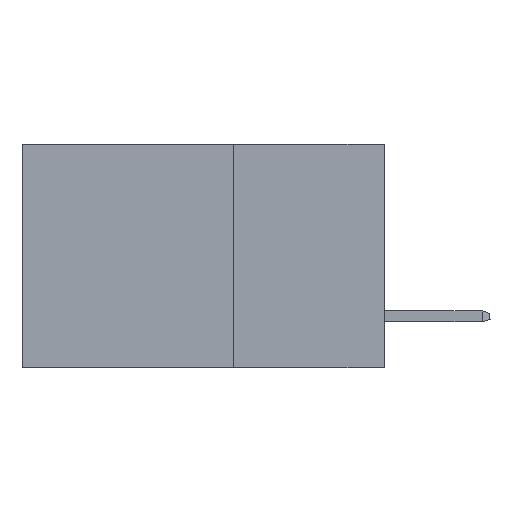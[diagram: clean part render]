
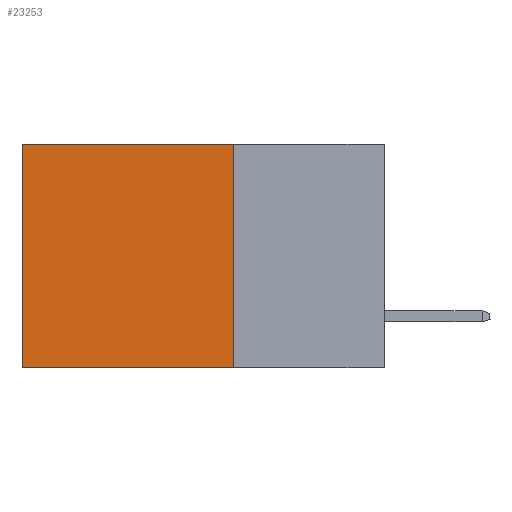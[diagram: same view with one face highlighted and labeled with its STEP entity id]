
A CAD part, left-side view. The second image highlights one B-rep face of the part: STEP entity #23253.
In plain terms, the highlighted planar face has unit normal (-1, 0, 0).
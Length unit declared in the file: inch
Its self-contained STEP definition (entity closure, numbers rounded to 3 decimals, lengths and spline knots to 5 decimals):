
#856 = CARTESIAN_POINT ( 'NONE',  ( 0.298, 0.6, 0. ) ) ;
#1150 = FACE_OUTER_BOUND ( 'NONE', #5787, .T. ) ;
#1282 = AXIS2_PLACEMENT_3D ( 'NONE', #12251, #8460, #14535 ) ;
#1731 = LINE ( 'NONE', #18426, #20809 ) ;
#4433 = VECTOR ( 'NONE', #16250, 39.37008 ) ;
#5022 = CARTESIAN_POINT ( 'NONE',  ( 0.298, 0.25, 0. ) ) ;
#5787 = EDGE_LOOP ( 'NONE', ( #23799, #16752, #11479, #19710 ) ) ;
#6522 = DIRECTION ( 'NONE',  ( 0., 0., -1. ) ) ;
#7714 = CARTESIAN_POINT ( 'NONE',  ( 0.298, 0.6, 0. ) ) ;
#8460 = DIRECTION ( 'NONE',  ( 1., 0., 0. ) ) ;
#8513 = LINE ( 'NONE', #856, #18653 ) ;
#8552 = VERTEX_POINT ( 'NONE', #15728 ) ;
#10761 = LINE ( 'NONE', #5022, #4433 ) ;
#11085 = CARTESIAN_POINT ( 'NONE',  ( 0.298, 0.25, 0. ) ) ;
#11275 = DIRECTION ( 'NONE',  ( 0., 0., -1. ) ) ;
#11479 = ORIENTED_EDGE ( 'NONE', *, *, #13270, .F. ) ;
#12226 = EDGE_CURVE ( 'NONE', #18486, #8552, #1731, .T. ) ;
#12251 = CARTESIAN_POINT ( 'NONE',  ( 0.298, 0.25, 0. ) ) ;
#12773 = VERTEX_POINT ( 'NONE', #7714 ) ;
#13270 = EDGE_CURVE ( 'NONE', #23477, #18486, #20190, .T. ) ;
#13540 = VECTOR ( 'NONE', #11275, 39.37008 ) ;
#14206 = PLANE ( 'NONE',  #1282 ) ;
#14535 = DIRECTION ( 'NONE',  ( 0., 0., -1. ) ) ;
#15475 = EDGE_CURVE ( 'NONE', #12773, #8552, #8513, .T. ) ;
#15728 = CARTESIAN_POINT ( 'NONE',  ( 0.298, 0.6, -0.37 ) ) ;
#16250 = DIRECTION ( 'NONE',  ( 0., 1., 0. ) ) ;
#16588 = DIRECTION ( 'NONE',  ( 0., 1., 0. ) ) ;
#16752 = ORIENTED_EDGE ( 'NONE', *, *, #12226, .F. ) ;
#16939 = CARTESIAN_POINT ( 'NONE',  ( 0.298, 0.25, -0.37 ) ) ;
#18426 = CARTESIAN_POINT ( 'NONE',  ( 0.298, 0.25, -0.37 ) ) ;
#18486 = VERTEX_POINT ( 'NONE', #16939 ) ;
#18653 = VECTOR ( 'NONE', #6522, 39.37008 ) ;
#19710 = ORIENTED_EDGE ( 'NONE', *, *, #21877, .T. ) ;
#20190 = LINE ( 'NONE', #20564, #13540 ) ;
#20564 = CARTESIAN_POINT ( 'NONE',  ( 0.298, 0.25, 0. ) ) ;
#20809 = VECTOR ( 'NONE', #16588, 39.37008 ) ;
#21877 = EDGE_CURVE ( 'NONE', #23477, #12773, #10761, .T. ) ;
#23253 = ADVANCED_FACE ( 'NONE', ( #1150 ), #14206, .F. ) ;
#23477 = VERTEX_POINT ( 'NONE', #11085 ) ;
#23799 = ORIENTED_EDGE ( 'NONE', *, *, #15475, .T. ) ;
